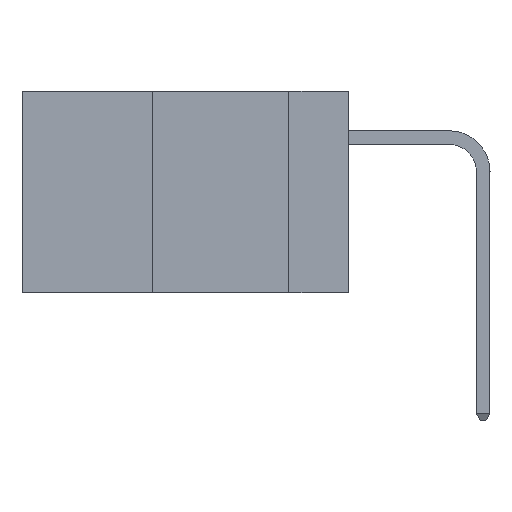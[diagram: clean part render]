
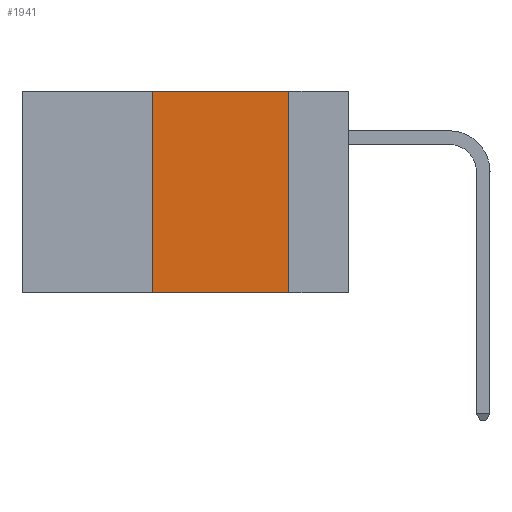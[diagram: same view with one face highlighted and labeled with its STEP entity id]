
A CAD part, left-side view. The second image highlights one B-rep face of the part: STEP entity #1941.
In plain terms, the highlighted planar face has unit normal (-1, 0, 0).
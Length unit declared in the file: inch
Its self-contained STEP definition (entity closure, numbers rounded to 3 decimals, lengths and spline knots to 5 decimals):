
#1941 = ADVANCED_FACE ( 'NONE', ( #19620 ), #22275, .F. ) ;
#2347 = EDGE_CURVE ( 'NONE', #13586, #19275, #11845, .T. ) ;
#2997 = ORIENTED_EDGE ( 'NONE', *, *, #2347, .F. ) ;
#3681 = EDGE_CURVE ( 'NONE', #8866, #6230, #4150, .T. ) ;
#3731 = ORIENTED_EDGE ( 'NONE', *, *, #4330, .F. ) ;
#4027 = ORIENTED_EDGE ( 'NONE', *, *, #3681, .F. ) ;
#4150 = LINE ( 'NONE', #18084, #23943 ) ;
#4330 = EDGE_CURVE ( 'NONE', #6230, #13586, #13517, .T. ) ;
#4726 = ORIENTED_EDGE ( 'NONE', *, *, #6318, .T. ) ;
#6230 = VERTEX_POINT ( 'NONE', #21120 ) ;
#6318 = EDGE_CURVE ( 'NONE', #8866, #19275, #20114, .T. ) ;
#8135 = VECTOR ( 'NONE', #21126, 39.37008 ) ;
#8866 = VERTEX_POINT ( 'NONE', #20986 ) ;
#9266 = AXIS2_PLACEMENT_3D ( 'NONE', #23212, #22114, #21835 ) ;
#9873 = CARTESIAN_POINT ( 'NONE',  ( 0., 0.6, -0.37 ) ) ;
#11845 = LINE ( 'NONE', #24093, #20752 ) ;
#13002 = CARTESIAN_POINT ( 'NONE',  ( 0., 0.11, -0.37 ) ) ;
#13517 = LINE ( 'NONE', #23036, #8135 ) ;
#13586 = VERTEX_POINT ( 'NONE', #19204 ) ;
#17601 = DIRECTION ( 'NONE',  ( 0., -1., 0. ) ) ;
#17917 = DIRECTION ( 'NONE',  ( 0., 0., 1. ) ) ;
#18084 = CARTESIAN_POINT ( 'NONE',  ( 0., 0.36, 0. ) ) ;
#19204 = CARTESIAN_POINT ( 'NONE',  ( 0., 0.11, 0. ) ) ;
#19275 = VERTEX_POINT ( 'NONE', #13002 ) ;
#19541 = VECTOR ( 'NONE', #17601, 39.37008 ) ;
#19620 = FACE_OUTER_BOUND ( 'NONE', #21283, .T. ) ;
#20114 = LINE ( 'NONE', #9873, #19541 ) ;
#20752 = VECTOR ( 'NONE', #24686, 39.37008 ) ;
#20986 = CARTESIAN_POINT ( 'NONE',  ( 0., 0.36, -0.37 ) ) ;
#21120 = CARTESIAN_POINT ( 'NONE',  ( 0., 0.36, 0. ) ) ;
#21126 = DIRECTION ( 'NONE',  ( 0., -1., 0. ) ) ;
#21283 = EDGE_LOOP ( 'NONE', ( #2997, #3731, #4027, #4726 ) ) ;
#21835 = DIRECTION ( 'NONE',  ( 0., 0., -1. ) ) ;
#22114 = DIRECTION ( 'NONE',  ( 1., 0., 0. ) ) ;
#22275 = PLANE ( 'NONE',  #9266 ) ;
#23036 = CARTESIAN_POINT ( 'NONE',  ( 0., 0.6, 0. ) ) ;
#23212 = CARTESIAN_POINT ( 'NONE',  ( 0., 0.6, 0. ) ) ;
#23943 = VECTOR ( 'NONE', #17917, 39.37008 ) ;
#24093 = CARTESIAN_POINT ( 'NONE',  ( 0., 0.11, 0. ) ) ;
#24686 = DIRECTION ( 'NONE',  ( 0., 0., -1. ) ) ;
